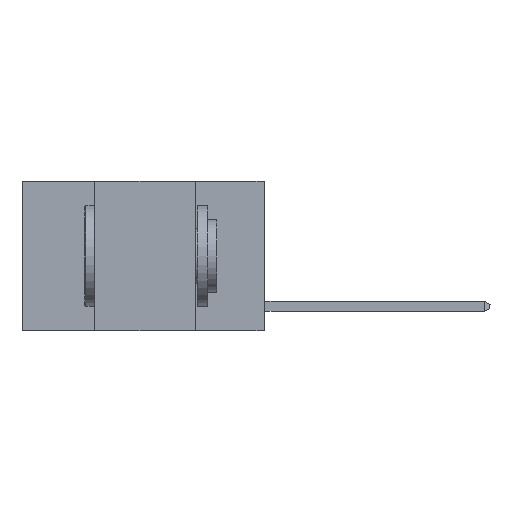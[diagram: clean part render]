
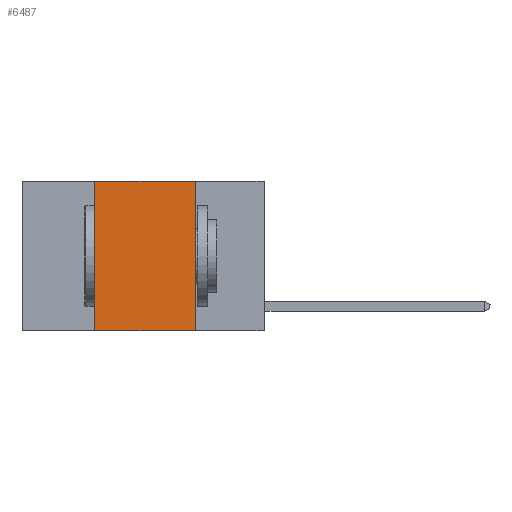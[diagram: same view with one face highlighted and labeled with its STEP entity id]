
A CAD part, left-side view. The second image highlights one B-rep face of the part: STEP entity #6487.
In plain terms, the highlighted planar face has unit normal (-1, 0, 0).
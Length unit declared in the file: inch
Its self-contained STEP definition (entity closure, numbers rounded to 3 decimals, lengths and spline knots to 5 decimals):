
#2013 = FACE_OUTER_BOUND ( 'NONE', #7665, .T. ) ;
#2120 = DIRECTION ( 'NONE',  ( 1., 0., 0. ) ) ;
#2215 = CARTESIAN_POINT ( 'NONE',  ( 0., 0.6, 0. ) ) ;
#2665 = EDGE_CURVE ( 'NONE', #3592, #25701, #16869, .T. ) ;
#3592 = VERTEX_POINT ( 'NONE', #11778 ) ;
#3752 = CARTESIAN_POINT ( 'NONE',  ( 0., 0.6, 0. ) ) ;
#4565 = DIRECTION ( 'NONE',  ( 0., 0., -1. ) ) ;
#6424 = CARTESIAN_POINT ( 'NONE',  ( 0., 0.17, -0.37 ) ) ;
#6487 = ADVANCED_FACE ( 'NONE', ( #2013 ), #18488, .F. ) ;
#6526 = ORIENTED_EDGE ( 'NONE', *, *, #23900, .F. ) ;
#7665 = EDGE_LOOP ( 'NONE', ( #7869, #15476, #6526, #8327 ) ) ;
#7869 = ORIENTED_EDGE ( 'NONE', *, *, #10619, .F. ) ;
#7914 = VERTEX_POINT ( 'NONE', #10833 ) ;
#8327 = ORIENTED_EDGE ( 'NONE', *, *, #2665, .T. ) ;
#10619 = EDGE_CURVE ( 'NONE', #7914, #25701, #21870, .T. ) ;
#10833 = CARTESIAN_POINT ( 'NONE',  ( 0., 0.17, 0. ) ) ;
#11522 = VERTEX_POINT ( 'NONE', #19736 ) ;
#11778 = CARTESIAN_POINT ( 'NONE',  ( 0., 0.42, -0.37 ) ) ;
#12632 = VECTOR ( 'NONE', #24943, 39.37008 ) ;
#12734 = DIRECTION ( 'NONE',  ( 0., 0., -1. ) ) ;
#14946 = LINE ( 'NONE', #25142, #12632 ) ;
#15465 = CARTESIAN_POINT ( 'NONE',  ( 0., 0.6, -0.37 ) ) ;
#15476 = ORIENTED_EDGE ( 'NONE', *, *, #23905, .F. ) ;
#15637 = DIRECTION ( 'NONE',  ( 0., -1., 0. ) ) ;
#16869 = LINE ( 'NONE', #15465, #17856 ) ;
#16897 = VECTOR ( 'NONE', #18925, 39.37008 ) ;
#17856 = VECTOR ( 'NONE', #15637, 39.37008 ) ;
#18488 = PLANE ( 'NONE',  #23300 ) ;
#18925 = DIRECTION ( 'NONE',  ( 0., -1., 0. ) ) ;
#19736 = CARTESIAN_POINT ( 'NONE',  ( 0., 0.42, 0. ) ) ;
#21062 = LINE ( 'NONE', #2215, #16897 ) ;
#21353 = CARTESIAN_POINT ( 'NONE',  ( 0., 0.17, 0. ) ) ;
#21870 = LINE ( 'NONE', #21353, #24733 ) ;
#23300 = AXIS2_PLACEMENT_3D ( 'NONE', #3752, #2120, #12734 ) ;
#23900 = EDGE_CURVE ( 'NONE', #3592, #11522, #14946, .T. ) ;
#23905 = EDGE_CURVE ( 'NONE', #11522, #7914, #21062, .T. ) ;
#24733 = VECTOR ( 'NONE', #4565, 39.37008 ) ;
#24943 = DIRECTION ( 'NONE',  ( 0., 0., 1. ) ) ;
#25142 = CARTESIAN_POINT ( 'NONE',  ( 0., 0.42, 0. ) ) ;
#25701 = VERTEX_POINT ( 'NONE', #6424 ) ;
